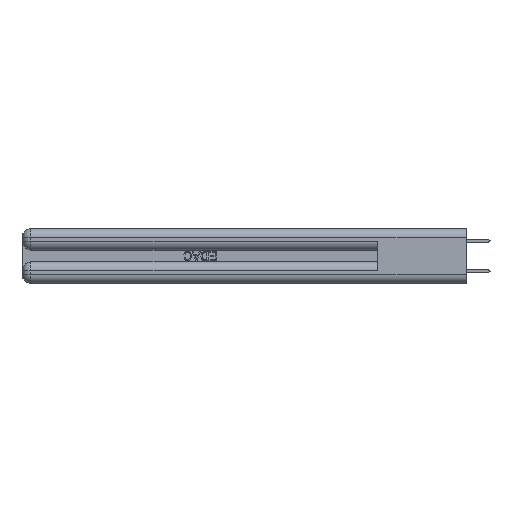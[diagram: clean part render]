
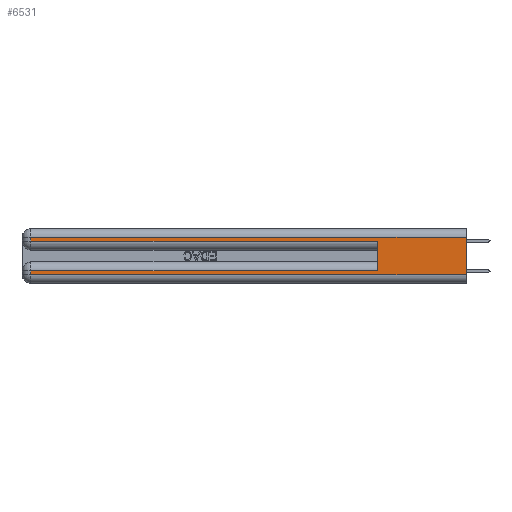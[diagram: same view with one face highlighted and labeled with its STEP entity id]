
A CAD part, left-side view. The second image highlights one B-rep face of the part: STEP entity #6531.
In plain terms, the highlighted planar face has unit normal (-1, 0, 0).
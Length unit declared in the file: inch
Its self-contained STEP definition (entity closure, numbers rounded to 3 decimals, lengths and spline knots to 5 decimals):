
#1212 = CARTESIAN_POINT ( 'NONE',  ( 0., 0.6, 0.145 ) ) ;
#1509 = DIRECTION ( 'NONE',  ( 0., 0., -1. ) ) ;
#2048 = LINE ( 'NONE', #20484, #43761 ) ;
#2148 = EDGE_CURVE ( 'NONE', #41370, #45001, #44964, .T. ) ;
#2523 = EDGE_CURVE ( 'NONE', #30746, #39983, #20706, .T. ) ;
#2927 = EDGE_CURVE ( 'NONE', #30746, #33932, #2048, .T. ) ;
#2948 = LINE ( 'NONE', #46157, #40097 ) ;
#3152 = ORIENTED_EDGE ( 'NONE', *, *, #19302, .F. ) ;
#3424 = DIRECTION ( 'NONE',  ( 0., 1., 0. ) ) ;
#4435 = LINE ( 'NONE', #44826, #8375 ) ;
#4928 = DIRECTION ( 'NONE',  ( 0., -1., 0. ) ) ;
#5598 = VERTEX_POINT ( 'NONE', #45243 ) ;
#6474 = VECTOR ( 'NONE', #4928, 39.37008 ) ;
#6531 = ADVANCED_FACE ( 'NONE', ( #45463 ), #19496, .F. ) ;
#8074 = EDGE_LOOP ( 'NONE', ( #3152, #35756, #26034, #21013, #9586, #33691, #33837, #26323 ) ) ;
#8375 = VECTOR ( 'NONE', #12251, 39.37008 ) ;
#9586 = ORIENTED_EDGE ( 'NONE', *, *, #2523, .F. ) ;
#10256 = DIRECTION ( 'NONE',  ( 0., 0., -1. ) ) ;
#10270 = DIRECTION ( 'NONE',  ( 0., 1., 0. ) ) ;
#11571 = CARTESIAN_POINT ( 'NONE',  ( 0., 0.6, 0.085 ) ) ;
#11716 = CARTESIAN_POINT ( 'NONE',  ( 0., 0., 0.06 ) ) ;
#11885 = CARTESIAN_POINT ( 'NONE',  ( 0., 2.94, 0.085 ) ) ;
#12251 = DIRECTION ( 'NONE',  ( 0., 0., -1. ) ) ;
#13261 = LINE ( 'NONE', #11716, #6474 ) ;
#13420 = CARTESIAN_POINT ( 'NONE',  ( 0., 0., 0.31 ) ) ;
#17312 = VECTOR ( 'NONE', #33192, 39.37008 ) ;
#19302 = EDGE_CURVE ( 'NONE', #41370, #5598, #2948, .T. ) ;
#19496 = PLANE ( 'NONE',  #26979 ) ;
#20484 = CARTESIAN_POINT ( 'NONE',  ( 0., 0., 0.085 ) ) ;
#20706 = LINE ( 'NONE', #1212, #17312 ) ;
#21013 = ORIENTED_EDGE ( 'NONE', *, *, #23831, .T. ) ;
#23831 = EDGE_CURVE ( 'NONE', #44366, #39983, #41728, .T. ) ;
#24724 = EDGE_CURVE ( 'NONE', #45001, #44366, #34112, .T. ) ;
#25056 = EDGE_CURVE ( 'NONE', #27251, #5598, #13261, .T. ) ;
#26034 = ORIENTED_EDGE ( 'NONE', *, *, #24724, .T. ) ;
#26323 = ORIENTED_EDGE ( 'NONE', *, *, #25056, .T. ) ;
#26396 = CARTESIAN_POINT ( 'NONE',  ( 0., 2.94, 0.31 ) ) ;
#26660 = CARTESIAN_POINT ( 'NONE',  ( 0., 0., 0.285 ) ) ;
#26979 = AXIS2_PLACEMENT_3D ( 'NONE', #40879, #33673, #1509 ) ;
#27251 = VERTEX_POINT ( 'NONE', #30886 ) ;
#30125 = DIRECTION ( 'NONE',  ( 0., -1., 0. ) ) ;
#30746 = VERTEX_POINT ( 'NONE', #11571 ) ;
#30872 = CARTESIAN_POINT ( 'NONE',  ( 0., 2.94, 0.285 ) ) ;
#30886 = CARTESIAN_POINT ( 'NONE',  ( 0., 2.94, 0.06 ) ) ;
#30897 = CARTESIAN_POINT ( 'NONE',  ( 0., 0., 0.31 ) ) ;
#32145 = VECTOR ( 'NONE', #30125, 39.37008 ) ;
#33192 = DIRECTION ( 'NONE',  ( 0., 0., 1. ) ) ;
#33673 = DIRECTION ( 'NONE',  ( 1., 0., 0. ) ) ;
#33691 = ORIENTED_EDGE ( 'NONE', *, *, #2927, .T. ) ;
#33837 = ORIENTED_EDGE ( 'NONE', *, *, #46371, .T. ) ;
#33932 = VERTEX_POINT ( 'NONE', #11885 ) ;
#34112 = LINE ( 'NONE', #41944, #36909 ) ;
#35756 = ORIENTED_EDGE ( 'NONE', *, *, #2148, .T. ) ;
#36909 = VECTOR ( 'NONE', #38514, 39.37008 ) ;
#37637 = VECTOR ( 'NONE', #10270, 39.37008 ) ;
#37757 = CARTESIAN_POINT ( 'NONE',  ( 0., 0.6, 0.285 ) ) ;
#38514 = DIRECTION ( 'NONE',  ( 0., 0., -1. ) ) ;
#39983 = VERTEX_POINT ( 'NONE', #37757 ) ;
#40097 = VECTOR ( 'NONE', #10256, 39.37008 ) ;
#40879 = CARTESIAN_POINT ( 'NONE',  ( 0., 0., 0.37 ) ) ;
#41370 = VERTEX_POINT ( 'NONE', #30897 ) ;
#41728 = LINE ( 'NONE', #26660, #32145 ) ;
#41944 = CARTESIAN_POINT ( 'NONE',  ( 0., 2.94, 0.37 ) ) ;
#43761 = VECTOR ( 'NONE', #3424, 39.37008 ) ;
#44366 = VERTEX_POINT ( 'NONE', #30872 ) ;
#44826 = CARTESIAN_POINT ( 'NONE',  ( 0., 2.94, 0.37 ) ) ;
#44964 = LINE ( 'NONE', #13420, #37637 ) ;
#45001 = VERTEX_POINT ( 'NONE', #26396 ) ;
#45243 = CARTESIAN_POINT ( 'NONE',  ( 0., 0., 0.06 ) ) ;
#45463 = FACE_OUTER_BOUND ( 'NONE', #8074, .T. ) ;
#46157 = CARTESIAN_POINT ( 'NONE',  ( 0., 0., 0.37 ) ) ;
#46371 = EDGE_CURVE ( 'NONE', #33932, #27251, #4435, .T. ) ;
